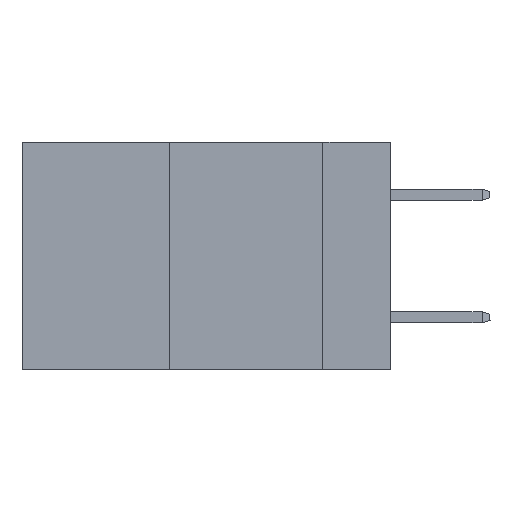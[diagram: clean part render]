
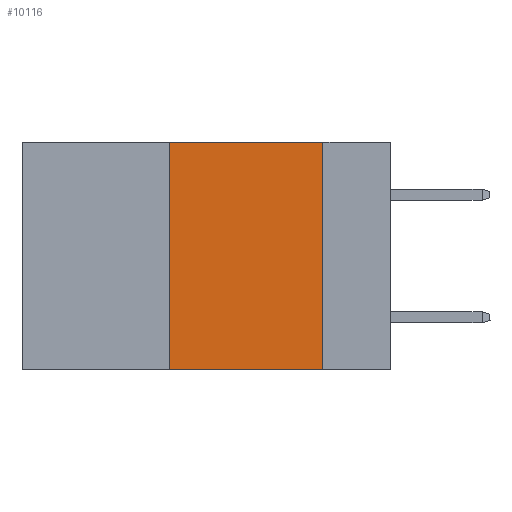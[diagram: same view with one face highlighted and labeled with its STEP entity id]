
A CAD part, left-side view. The second image highlights one B-rep face of the part: STEP entity #10116.
In plain terms, the highlighted planar face has unit normal (-1, 0, 0).
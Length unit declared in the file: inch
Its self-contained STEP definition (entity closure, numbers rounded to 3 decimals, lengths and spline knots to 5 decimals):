
#1089 = CARTESIAN_POINT ( 'NONE',  ( 0., 0.6, -0.37 ) ) ;
#1095 = DIRECTION ( 'NONE',  ( 0., -1., 0. ) ) ;
#2413 = DIRECTION ( 'NONE',  ( 0., -1., 0. ) ) ;
#2450 = LINE ( 'NONE', #15674, #13003 ) ;
#2811 = CARTESIAN_POINT ( 'NONE',  ( 0., 0.6, 0. ) ) ;
#3173 = CARTESIAN_POINT ( 'NONE',  ( 0., 0.11, 0. ) ) ;
#4182 = LINE ( 'NONE', #1089, #12212 ) ;
#4411 = DIRECTION ( 'NONE',  ( 0., 0., -1. ) ) ;
#4606 = ORIENTED_EDGE ( 'NONE', *, *, #10728, .F. ) ;
#5480 = FACE_OUTER_BOUND ( 'NONE', #18923, .T. ) ;
#5677 = ORIENTED_EDGE ( 'NONE', *, *, #12120, .F. ) ;
#5892 = PLANE ( 'NONE',  #6361 ) ;
#6361 = AXIS2_PLACEMENT_3D ( 'NONE', #2811, #15759, #4411 ) ;
#7461 = VECTOR ( 'NONE', #9876, 39.37008 ) ;
#7932 = VERTEX_POINT ( 'NONE', #14064 ) ;
#9876 = DIRECTION ( 'NONE',  ( 0., 0., -1. ) ) ;
#10116 = ADVANCED_FACE ( 'NONE', ( #5480 ), #5892, .F. ) ;
#10728 = EDGE_CURVE ( 'NONE', #18600, #7932, #20033, .T. ) ;
#10811 = ORIENTED_EDGE ( 'NONE', *, *, #17591, .F. ) ;
#12088 = CARTESIAN_POINT ( 'NONE',  ( 0., 0.6, 0. ) ) ;
#12120 = EDGE_CURVE ( 'NONE', #17867, #18600, #18491, .T. ) ;
#12212 = VECTOR ( 'NONE', #2413, 39.37008 ) ;
#13003 = VECTOR ( 'NONE', #18825, 39.37008 ) ;
#14064 = CARTESIAN_POINT ( 'NONE',  ( 0., 0.11, -0.37 ) ) ;
#15674 = CARTESIAN_POINT ( 'NONE',  ( 0., 0.36, 0. ) ) ;
#15759 = DIRECTION ( 'NONE',  ( 1., 0., 0. ) ) ;
#16134 = CARTESIAN_POINT ( 'NONE',  ( 0., 0.11, 0. ) ) ;
#16701 = CARTESIAN_POINT ( 'NONE',  ( 0., 0.36, 0. ) ) ;
#17591 = EDGE_CURVE ( 'NONE', #17729, #17867, #2450, .T. ) ;
#17729 = VERTEX_POINT ( 'NONE', #18981 ) ;
#17783 = ORIENTED_EDGE ( 'NONE', *, *, #19016, .T. ) ;
#17867 = VERTEX_POINT ( 'NONE', #16701 ) ;
#17954 = VECTOR ( 'NONE', #1095, 39.37008 ) ;
#18491 = LINE ( 'NONE', #12088, #17954 ) ;
#18600 = VERTEX_POINT ( 'NONE', #3173 ) ;
#18825 = DIRECTION ( 'NONE',  ( 0., 0., 1. ) ) ;
#18923 = EDGE_LOOP ( 'NONE', ( #4606, #5677, #10811, #17783 ) ) ;
#18981 = CARTESIAN_POINT ( 'NONE',  ( 0., 0.36, -0.37 ) ) ;
#19016 = EDGE_CURVE ( 'NONE', #17729, #7932, #4182, .T. ) ;
#20033 = LINE ( 'NONE', #16134, #7461 ) ;
